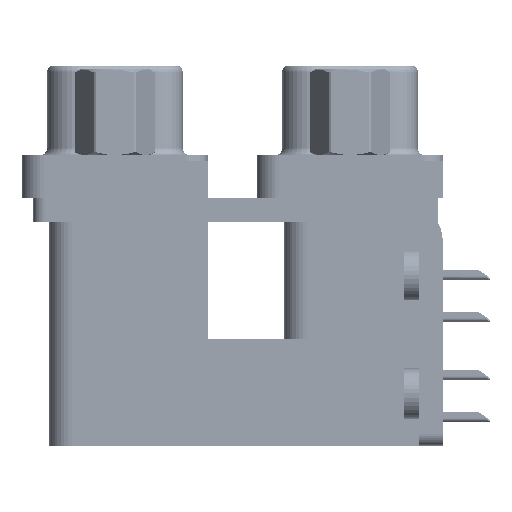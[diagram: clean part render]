
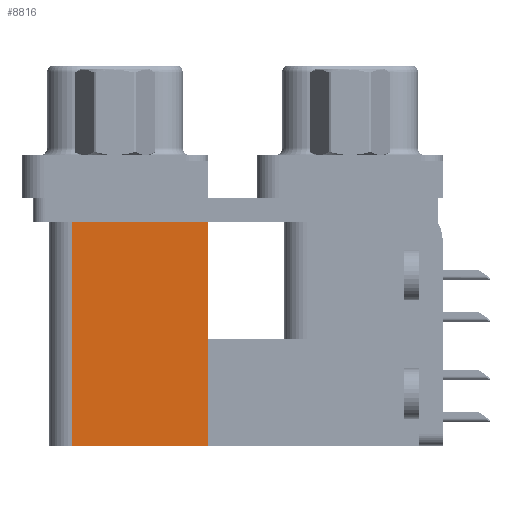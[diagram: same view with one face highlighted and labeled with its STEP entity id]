
A CAD part, left-side view. The second image highlights one B-rep face of the part: STEP entity #8816.
In plain terms, the highlighted planar face has unit normal (-1, 0, 0).
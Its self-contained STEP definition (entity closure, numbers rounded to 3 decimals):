
#1333 = ORIENTED_EDGE ( 'NONE', *, *, #37662, .F. ) ;
#1939 = FACE_OUTER_BOUND ( 'NONE', #4097, .T. ) ;
#2182 = CARTESIAN_POINT ( 'NONE',  ( 3.7, 9.6, -19.2 ) ) ;
#3411 = LINE ( 'NONE', #18105, #17733 ) ;
#3879 = LINE ( 'NONE', #45073, #5036 ) ;
#4097 = EDGE_LOOP ( 'NONE', ( #43627, #1333, #37572, #29382 ) ) ;
#5036 = VECTOR ( 'NONE', #22427, 1000. ) ;
#6496 = DIRECTION ( 'NONE',  ( 1., 0., 0. ) ) ;
#8633 = EDGE_CURVE ( 'NONE', #43934, #22712, #3411, .T. ) ;
#8816 = ADVANCED_FACE ( 'NONE', ( #1939 ), #9873, .F. ) ;
#9873 = PLANE ( 'NONE',  #47060 ) ;
#12112 = CARTESIAN_POINT ( 'NONE',  ( 3.7, 9.6, -2.5 ) ) ;
#17198 = CARTESIAN_POINT ( 'NONE',  ( 3.7, 9.6, -2.5 ) ) ;
#17733 = VECTOR ( 'NONE', #43878, 1000. ) ;
#17903 = LINE ( 'NONE', #17198, #29779 ) ;
#18105 = CARTESIAN_POINT ( 'NONE',  ( 3.7, 9.6, -19.2 ) ) ;
#18343 = CARTESIAN_POINT ( 'NONE',  ( 3.7, 18.8, -2.5 ) ) ;
#20533 = CARTESIAN_POINT ( 'NONE',  ( 3.7, 18.8, -19.2 ) ) ;
#22427 = DIRECTION ( 'NONE',  ( 0., 0., 1. ) ) ;
#22712 = VERTEX_POINT ( 'NONE', #24922 ) ;
#23651 = DIRECTION ( 'NONE',  ( 0., 0., 1. ) ) ;
#24922 = CARTESIAN_POINT ( 'NONE',  ( 3.7, 18.8, -19.2 ) ) ;
#27303 = VERTEX_POINT ( 'NONE', #18343 ) ;
#29382 = ORIENTED_EDGE ( 'NONE', *, *, #40609, .T. ) ;
#29779 = VECTOR ( 'NONE', #32813, 1000. ) ;
#30929 = VERTEX_POINT ( 'NONE', #12112 ) ;
#32813 = DIRECTION ( 'NONE',  ( 0., 1., 0. ) ) ;
#37572 = ORIENTED_EDGE ( 'NONE', *, *, #8633, .F. ) ;
#37662 = EDGE_CURVE ( 'NONE', #22712, #27303, #41510, .T. ) ;
#39515 = DIRECTION ( 'NONE',  ( 0., 0., -1. ) ) ;
#40392 = CARTESIAN_POINT ( 'NONE',  ( 3.7, 9.6, -19.2 ) ) ;
#40609 = EDGE_CURVE ( 'NONE', #43934, #30929, #3879, .T. ) ;
#41510 = LINE ( 'NONE', #20533, #44849 ) ;
#43005 = EDGE_CURVE ( 'NONE', #30929, #27303, #17903, .T. ) ;
#43627 = ORIENTED_EDGE ( 'NONE', *, *, #43005, .T. ) ;
#43878 = DIRECTION ( 'NONE',  ( 0., 1., 0. ) ) ;
#43934 = VERTEX_POINT ( 'NONE', #40392 ) ;
#44849 = VECTOR ( 'NONE', #23651, 1000. ) ;
#45073 = CARTESIAN_POINT ( 'NONE',  ( 3.7, 9.6, -19.2 ) ) ;
#47060 = AXIS2_PLACEMENT_3D ( 'NONE', #2182, #6496, #39515 ) ;
